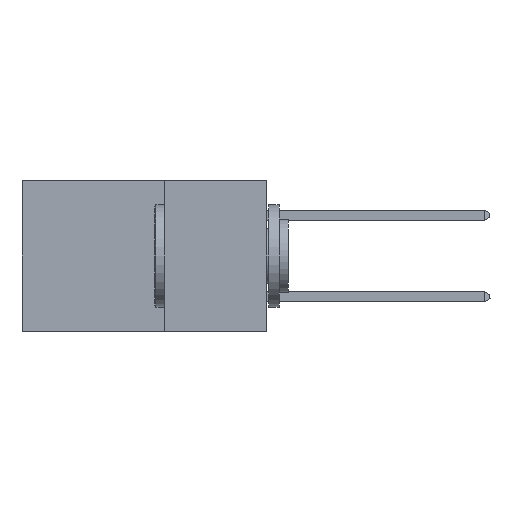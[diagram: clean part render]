
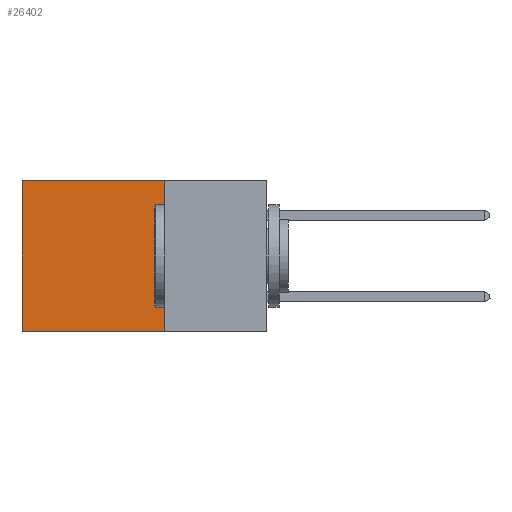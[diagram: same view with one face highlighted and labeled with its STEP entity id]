
A CAD part, left-side view. The second image highlights one B-rep face of the part: STEP entity #26402.
In plain terms, the highlighted planar face has unit normal (-1, 0, 0).
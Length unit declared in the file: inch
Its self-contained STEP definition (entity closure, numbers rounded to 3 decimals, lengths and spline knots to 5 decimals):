
#78 = LINE ( 'NONE', #21860, #19224 ) ;
#737 = VECTOR ( 'NONE', #6895, 39.37008 ) ;
#1165 = CARTESIAN_POINT ( 'NONE',  ( 0.2875, 0.25, -0.37 ) ) ;
#3371 = CARTESIAN_POINT ( 'NONE',  ( 0.2875, 0.6, -0.37 ) ) ;
#3866 = CARTESIAN_POINT ( 'NONE',  ( 0.2875, 0.25, -0.37 ) ) ;
#4496 = CARTESIAN_POINT ( 'NONE',  ( 0.2875, 0.25, 0. ) ) ;
#4777 = VECTOR ( 'NONE', #8599, 39.37008 ) ;
#4850 = VERTEX_POINT ( 'NONE', #4496 ) ;
#5276 = CARTESIAN_POINT ( 'NONE',  ( 0.2875, 0.6, 0. ) ) ;
#5641 = LINE ( 'NONE', #3866, #27613 ) ;
#5653 = ORIENTED_EDGE ( 'NONE', *, *, #8096, .F. ) ;
#6895 = DIRECTION ( 'NONE',  ( 0., 0., -1. ) ) ;
#7681 = EDGE_LOOP ( 'NONE', ( #23304, #7880, #5653, #13346 ) ) ;
#7880 = ORIENTED_EDGE ( 'NONE', *, *, #24785, .F. ) ;
#8096 = EDGE_CURVE ( 'NONE', #4850, #21262, #27807, .T. ) ;
#8599 = DIRECTION ( 'NONE',  ( 0., 0., -1. ) ) ;
#11954 = VERTEX_POINT ( 'NONE', #5276 ) ;
#13262 = CARTESIAN_POINT ( 'NONE',  ( 0.2875, 0.25, 0. ) ) ;
#13346 = ORIENTED_EDGE ( 'NONE', *, *, #29941, .T. ) ;
#14350 = CARTESIAN_POINT ( 'NONE',  ( 0.2875, 0.25, 0. ) ) ;
#18898 = EDGE_CURVE ( 'NONE', #11954, #26094, #25110, .T. ) ;
#19224 = VECTOR ( 'NONE', #24473, 39.37008 ) ;
#20949 = CARTESIAN_POINT ( 'NONE',  ( 0.2875, 0.6, 0. ) ) ;
#21262 = VERTEX_POINT ( 'NONE', #1165 ) ;
#21377 = DIRECTION ( 'NONE',  ( 0., 1., 0. ) ) ;
#21860 = CARTESIAN_POINT ( 'NONE',  ( 0.2875, 0.25, 0. ) ) ;
#22490 = AXIS2_PLACEMENT_3D ( 'NONE', #13262, #23414, #25926 ) ;
#23304 = ORIENTED_EDGE ( 'NONE', *, *, #18898, .T. ) ;
#23414 = DIRECTION ( 'NONE',  ( 1., 0., 0. ) ) ;
#23587 = FACE_OUTER_BOUND ( 'NONE', #7681, .T. ) ;
#24473 = DIRECTION ( 'NONE',  ( 0., 1., 0. ) ) ;
#24785 = EDGE_CURVE ( 'NONE', #21262, #26094, #5641, .T. ) ;
#25110 = LINE ( 'NONE', #20949, #4777 ) ;
#25926 = DIRECTION ( 'NONE',  ( 0., 0., -1. ) ) ;
#26094 = VERTEX_POINT ( 'NONE', #3371 ) ;
#26402 = ADVANCED_FACE ( 'NONE', ( #23587 ), #27826, .F. ) ;
#27613 = VECTOR ( 'NONE', #21377, 39.37008 ) ;
#27807 = LINE ( 'NONE', #14350, #737 ) ;
#27826 = PLANE ( 'NONE',  #22490 ) ;
#29941 = EDGE_CURVE ( 'NONE', #4850, #11954, #78, .T. ) ;
